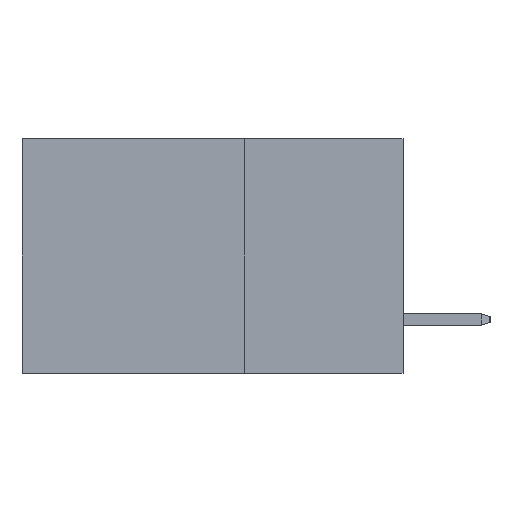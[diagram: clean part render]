
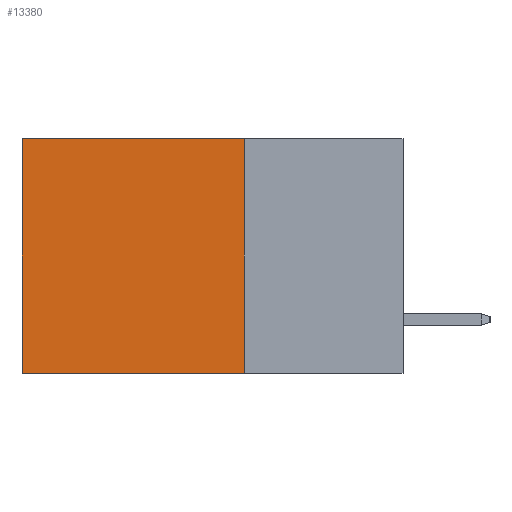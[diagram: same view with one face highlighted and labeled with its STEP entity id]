
A CAD part, left-side view. The second image highlights one B-rep face of the part: STEP entity #13380.
In plain terms, the highlighted planar face has unit normal (-1, 0, 0).
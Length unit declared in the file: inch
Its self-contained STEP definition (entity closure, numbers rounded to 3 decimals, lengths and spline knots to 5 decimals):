
#181 = EDGE_LOOP ( 'NONE', ( #2776, #8423, #9774, #14542 ) ) ;
#1330 = EDGE_CURVE ( 'NONE', #8584, #4124, #3592, .T. ) ;
#1677 = FACE_OUTER_BOUND ( 'NONE', #181, .T. ) ;
#2038 = DIRECTION ( 'NONE',  ( 0., 0., -1. ) ) ;
#2497 = CARTESIAN_POINT ( 'NONE',  ( 0.2875, 0.6, 0. ) ) ;
#2572 = VECTOR ( 'NONE', #4481, 39.37008 ) ;
#2776 = ORIENTED_EDGE ( 'NONE', *, *, #10839, .T. ) ;
#2856 = CARTESIAN_POINT ( 'NONE',  ( 0.2875, 0.25, -0.37 ) ) ;
#3352 = VERTEX_POINT ( 'NONE', #2856 ) ;
#3355 = CARTESIAN_POINT ( 'NONE',  ( 0.2875, 0.6, -0.37 ) ) ;
#3592 = LINE ( 'NONE', #8626, #3909 ) ;
#3909 = VECTOR ( 'NONE', #9957, 39.37008 ) ;
#4124 = VERTEX_POINT ( 'NONE', #2497 ) ;
#4481 = DIRECTION ( 'NONE',  ( 0., 0., -1. ) ) ;
#5135 = EDGE_CURVE ( 'NONE', #8584, #3352, #7935, .T. ) ;
#5136 = CARTESIAN_POINT ( 'NONE',  ( 0.2875, 0.25, 0. ) ) ;
#5366 = PLANE ( 'NONE',  #7458 ) ;
#5547 = CARTESIAN_POINT ( 'NONE',  ( 0.2875, 0.25, 0. ) ) ;
#5560 = CARTESIAN_POINT ( 'NONE',  ( 0.2875, 0.25, -0.37 ) ) ;
#7458 = AXIS2_PLACEMENT_3D ( 'NONE', #10062, #12613, #8323 ) ;
#7935 = LINE ( 'NONE', #5547, #2572 ) ;
#8323 = DIRECTION ( 'NONE',  ( 0., 0., -1. ) ) ;
#8423 = ORIENTED_EDGE ( 'NONE', *, *, #11239, .F. ) ;
#8584 = VERTEX_POINT ( 'NONE', #5136 ) ;
#8626 = CARTESIAN_POINT ( 'NONE',  ( 0.2875, 0.25, 0. ) ) ;
#9774 = ORIENTED_EDGE ( 'NONE', *, *, #5135, .F. ) ;
#9957 = DIRECTION ( 'NONE',  ( 0., 1., 0. ) ) ;
#10062 = CARTESIAN_POINT ( 'NONE',  ( 0.2875, 0.25, 0. ) ) ;
#10498 = LINE ( 'NONE', #5560, #11974 ) ;
#10839 = EDGE_CURVE ( 'NONE', #4124, #13979, #13062, .T. ) ;
#11239 = EDGE_CURVE ( 'NONE', #3352, #13979, #10498, .T. ) ;
#11974 = VECTOR ( 'NONE', #15671, 39.37008 ) ;
#12613 = DIRECTION ( 'NONE',  ( 1., 0., 0. ) ) ;
#12951 = VECTOR ( 'NONE', #2038, 39.37008 ) ;
#13062 = LINE ( 'NONE', #14535, #12951 ) ;
#13380 = ADVANCED_FACE ( 'NONE', ( #1677 ), #5366, .F. ) ;
#13979 = VERTEX_POINT ( 'NONE', #3355 ) ;
#14535 = CARTESIAN_POINT ( 'NONE',  ( 0.2875, 0.6, 0. ) ) ;
#14542 = ORIENTED_EDGE ( 'NONE', *, *, #1330, .T. ) ;
#15671 = DIRECTION ( 'NONE',  ( 0., 1., 0. ) ) ;
